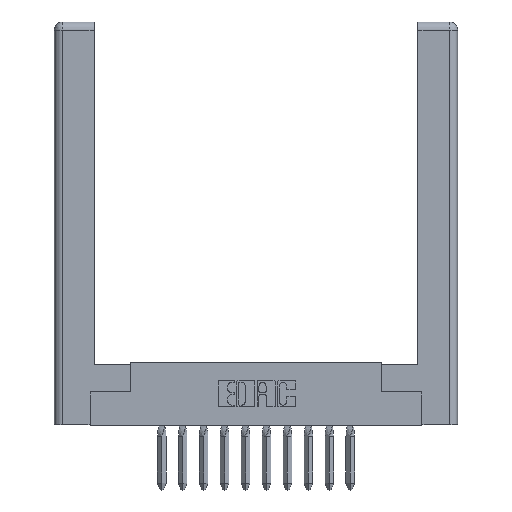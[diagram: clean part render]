
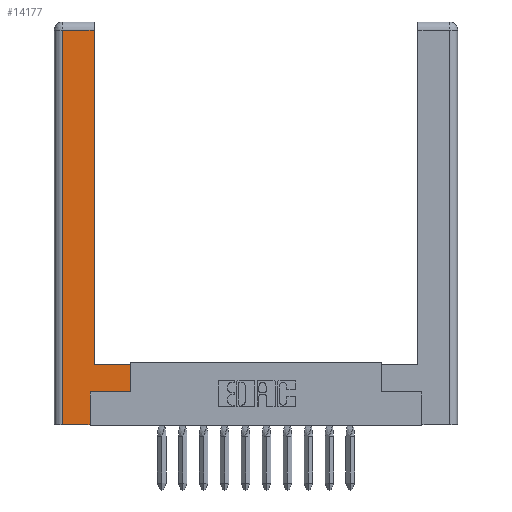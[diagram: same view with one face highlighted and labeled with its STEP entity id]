
A CAD part, top view. The second image highlights one B-rep face of the part: STEP entity #14177.
In plain terms, the highlighted planar face has unit normal (0, 0, 1).
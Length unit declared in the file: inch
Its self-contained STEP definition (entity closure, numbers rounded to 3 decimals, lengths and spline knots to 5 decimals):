
#85 = CARTESIAN_POINT ( 'NONE',  ( 0.0615, 0., 0. ) ) ;
#136 = VECTOR ( 'NONE', #14699, 39.37008 ) ;
#170 = EDGE_CURVE ( 'NONE', #21644, #2785, #2891, .T. ) ;
#1563 = DIRECTION ( 'NONE',  ( 0., 1., 0. ) ) ;
#2580 = DIRECTION ( 'NONE',  ( 0., 1., 0. ) ) ;
#2771 = LINE ( 'NONE', #25157, #4611 ) ;
#2785 = VERTEX_POINT ( 'NONE', #19944 ) ;
#2891 = LINE ( 'NONE', #24037, #9597 ) ;
#3012 = EDGE_CURVE ( 'NONE', #6677, #22513, #2771, .T. ) ;
#3592 = PLANE ( 'NONE',  #23737 ) ;
#3634 = VERTEX_POINT ( 'NONE', #21368 ) ;
#3838 = CARTESIAN_POINT ( 'NONE',  ( 0.265, 0., 0. ) ) ;
#3917 = CARTESIAN_POINT ( 'NONE',  ( 0.0615, 0., 0. ) ) ;
#4126 = CARTESIAN_POINT ( 'NONE',  ( 0.295, 3., 0. ) ) ;
#4611 = VECTOR ( 'NONE', #1563, 39.37008 ) ;
#5195 = VERTEX_POINT ( 'NONE', #19851 ) ;
#5679 = DIRECTION ( 'NONE',  ( -1., 0., 0. ) ) ;
#6082 = DIRECTION ( 'NONE',  ( 0., 1., 0. ) ) ;
#6168 = FACE_OUTER_BOUND ( 'NONE', #22174, .T. ) ;
#6342 = CARTESIAN_POINT ( 'NONE',  ( 0.0615, 2.94, 0. ) ) ;
#6658 = VECTOR ( 'NONE', #17240, 39.37008 ) ;
#6677 = VERTEX_POINT ( 'NONE', #20709 ) ;
#7110 = ORIENTED_EDGE ( 'NONE', *, *, #22741, .T. ) ;
#7320 = ORIENTED_EDGE ( 'NONE', *, *, #21587, .T. ) ;
#8433 = EDGE_CURVE ( 'NONE', #2785, #6677, #23407, .T. ) ;
#9597 = VECTOR ( 'NONE', #2580, 39.37008 ) ;
#9740 = CARTESIAN_POINT ( 'NONE',  ( 0.565, 0.245, 0. ) ) ;
#10262 = VECTOR ( 'NONE', #11348, 39.37008 ) ;
#10703 = ORIENTED_EDGE ( 'NONE', *, *, #16386, .T. ) ;
#11118 = VERTEX_POINT ( 'NONE', #85 ) ;
#11348 = DIRECTION ( 'NONE',  ( 1., 0., 0. ) ) ;
#11803 = VECTOR ( 'NONE', #6082, 39.37008 ) ;
#11856 = ORIENTED_EDGE ( 'NONE', *, *, #24822, .T. ) ;
#11912 = VERTEX_POINT ( 'NONE', #6342 ) ;
#12222 = VECTOR ( 'NONE', #5679, 39.37008 ) ;
#12719 = CARTESIAN_POINT ( 'NONE',  ( 0.295, 0.45, 0. ) ) ;
#12933 = ORIENTED_EDGE ( 'NONE', *, *, #3012, .T. ) ;
#13312 = CARTESIAN_POINT ( 'NONE',  ( 0.265, 0., 0. ) ) ;
#14177 = ADVANCED_FACE ( 'NONE', ( #6168 ), #3592, .F. ) ;
#14699 = DIRECTION ( 'NONE',  ( -1., 0., 0. ) ) ;
#15138 = CARTESIAN_POINT ( 'NONE',  ( 0.0615, 2.94, 0. ) ) ;
#15183 = CARTESIAN_POINT ( 'NONE',  ( 0., 0., 0. ) ) ;
#15486 = LINE ( 'NONE', #3917, #23098 ) ;
#15919 = ORIENTED_EDGE ( 'NONE', *, *, #8433, .T. ) ;
#16386 = EDGE_CURVE ( 'NONE', #5195, #3634, #17007, .T. ) ;
#17007 = LINE ( 'NONE', #4126, #11803 ) ;
#17240 = DIRECTION ( 'NONE',  ( 1., 0., 0. ) ) ;
#17416 = LINE ( 'NONE', #15138, #12222 ) ;
#18159 = LINE ( 'NONE', #13312, #10262 ) ;
#18680 = ORIENTED_EDGE ( 'NONE', *, *, #170, .T. ) ;
#18786 = ORIENTED_EDGE ( 'NONE', *, *, #20071, .T. ) ;
#19082 = DIRECTION ( 'NONE',  ( 0., 0., -1. ) ) ;
#19851 = CARTESIAN_POINT ( 'NONE',  ( 0.295, 0.45, 0. ) ) ;
#19944 = CARTESIAN_POINT ( 'NONE',  ( 0.265, 0.245, 0. ) ) ;
#19948 = LINE ( 'NONE', #12719, #136 ) ;
#20071 = EDGE_CURVE ( 'NONE', #3634, #11912, #17416, .T. ) ;
#20709 = CARTESIAN_POINT ( 'NONE',  ( 0.565, 0.245, 0. ) ) ;
#21142 = DIRECTION ( 'NONE',  ( 0., -1., 0. ) ) ;
#21368 = CARTESIAN_POINT ( 'NONE',  ( 0.295, 2.94, 0. ) ) ;
#21587 = EDGE_CURVE ( 'NONE', #11912, #11118, #15486, .T. ) ;
#21644 = VERTEX_POINT ( 'NONE', #3838 ) ;
#22174 = EDGE_LOOP ( 'NONE', ( #10703, #18786, #7320, #7110, #18680, #15919, #12933, #11856 ) ) ;
#22446 = CARTESIAN_POINT ( 'NONE',  ( 0.565, 0.45, 0. ) ) ;
#22513 = VERTEX_POINT ( 'NONE', #22446 ) ;
#22741 = EDGE_CURVE ( 'NONE', #11118, #21644, #18159, .T. ) ;
#23098 = VECTOR ( 'NONE', #21142, 39.37008 ) ;
#23261 = DIRECTION ( 'NONE',  ( -1., 0., 0. ) ) ;
#23407 = LINE ( 'NONE', #9740, #6658 ) ;
#23737 = AXIS2_PLACEMENT_3D ( 'NONE', #15183, #19082, #23261 ) ;
#24037 = CARTESIAN_POINT ( 'NONE',  ( 0.265, 0.245, 0. ) ) ;
#24822 = EDGE_CURVE ( 'NONE', #22513, #5195, #19948, .T. ) ;
#25157 = CARTESIAN_POINT ( 'NONE',  ( 0.565, 0.45, 0. ) ) ;
